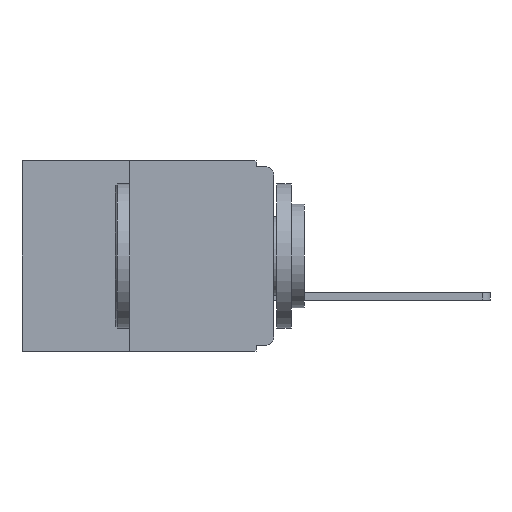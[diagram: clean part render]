
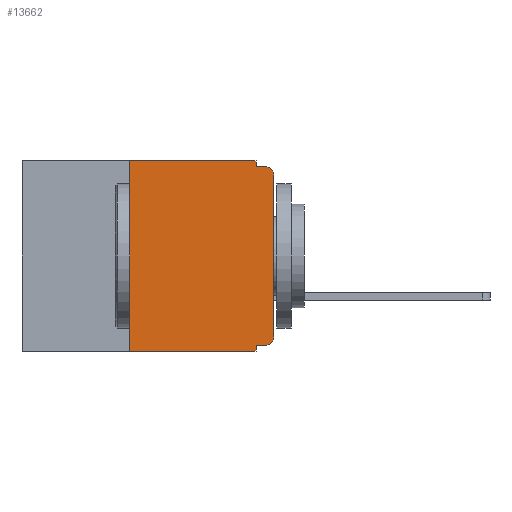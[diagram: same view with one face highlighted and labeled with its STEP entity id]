
A CAD part, left-side view. The second image highlights one B-rep face of the part: STEP entity #13662.
In plain terms, the highlighted planar face has unit normal (-1, 0, 0).
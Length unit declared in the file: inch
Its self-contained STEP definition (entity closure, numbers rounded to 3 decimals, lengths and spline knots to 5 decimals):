
#627 = CARTESIAN_POINT ( 'NONE',  ( 0., 0.031, 0. ) ) ;
#787 = ORIENTED_EDGE ( 'NONE', *, *, #3188, .F. ) ;
#835 = VECTOR ( 'NONE', #8509, 39.37008 ) ;
#1002 = DIRECTION ( 'NONE',  ( 0., 0., 1. ) ) ;
#1035 = CARTESIAN_POINT ( 'NONE',  ( 0., 0.25, 0. ) ) ;
#1057 = VECTOR ( 'NONE', #4462, 39.37008 ) ;
#1366 = CARTESIAN_POINT ( 'NONE',  ( 0., 0., -0.305 ) ) ;
#1656 = CARTESIAN_POINT ( 'NONE',  ( 0., 0.25, -0.33 ) ) ;
#2349 = CARTESIAN_POINT ( 'NONE',  ( 0., 0.031, -0.32 ) ) ;
#2461 = EDGE_CURVE ( 'NONE', #2758, #8635, #11873, .T. ) ;
#2539 = ORIENTED_EDGE ( 'NONE', *, *, #2461, .T. ) ;
#2572 = EDGE_CURVE ( 'NONE', #6670, #8470, #6861, .T. ) ;
#2703 = VERTEX_POINT ( 'NONE', #13685 ) ;
#2758 = VERTEX_POINT ( 'NONE', #6891 ) ;
#2934 = PLANE ( 'NONE',  #12298 ) ;
#3059 = EDGE_CURVE ( 'NONE', #6110, #9530, #4142, .T. ) ;
#3188 = EDGE_CURVE ( 'NONE', #2758, #6728, #3935, .T. ) ;
#3466 = EDGE_CURVE ( 'NONE', #2703, #6555, #9081, .T. ) ;
#3590 = EDGE_CURVE ( 'NONE', #10843, #6110, #10509, .T. ) ;
#3658 = AXIS2_PLACEMENT_3D ( 'NONE', #7960, #7852, #7808 ) ;
#3788 = EDGE_CURVE ( 'NONE', #8470, #9530, #9719, .T. ) ;
#3797 = ORIENTED_EDGE ( 'NONE', *, *, #4057, .F. ) ;
#3935 = LINE ( 'NONE', #1656, #12425 ) ;
#3991 = ORIENTED_EDGE ( 'NONE', *, *, #3466, .F. ) ;
#4057 = EDGE_CURVE ( 'NONE', #6555, #8635, #12536, .T. ) ;
#4110 = DIRECTION ( 'NONE',  ( 1., 0., 0. ) ) ;
#4142 = LINE ( 'NONE', #4792, #7203 ) ;
#4197 = DIRECTION ( 'NONE',  ( 0., -1., 0. ) ) ;
#4209 = EDGE_CURVE ( 'NONE', #2703, #6670, #4679, .T. ) ;
#4229 = ORIENTED_EDGE ( 'NONE', *, *, #4209, .T. ) ;
#4462 = DIRECTION ( 'NONE',  ( 0., 0., -1. ) ) ;
#4679 = CIRCLE ( 'NONE', #8775, 0.015 ) ;
#4792 = CARTESIAN_POINT ( 'NONE',  ( 0., 0., -0.01 ) ) ;
#5159 = ORIENTED_EDGE ( 'NONE', *, *, #3788, .T. ) ;
#5355 = LINE ( 'NONE', #10826, #10720 ) ;
#5729 = EDGE_CURVE ( 'NONE', #6728, #10843, #5355, .T. ) ;
#5818 = VECTOR ( 'NONE', #6712, 39.37008 ) ;
#6037 = DIRECTION ( 'NONE',  ( 0., 0., 1. ) ) ;
#6110 = VERTEX_POINT ( 'NONE', #6798 ) ;
#6408 = ORIENTED_EDGE ( 'NONE', *, *, #3059, .F. ) ;
#6555 = VERTEX_POINT ( 'NONE', #2349 ) ;
#6636 = CARTESIAN_POINT ( 'NONE',  ( 0., 0.031, -0.33 ) ) ;
#6651 = CARTESIAN_POINT ( 'NONE',  ( 0., 0., -0.32 ) ) ;
#6670 = VERTEX_POINT ( 'NONE', #1366 ) ;
#6712 = DIRECTION ( 'NONE',  ( 0., 1., 0. ) ) ;
#6728 = VERTEX_POINT ( 'NONE', #1035 ) ;
#6798 = CARTESIAN_POINT ( 'NONE',  ( 0., 0.031, -0.01 ) ) ;
#6861 = LINE ( 'NONE', #12198, #12288 ) ;
#6891 = CARTESIAN_POINT ( 'NONE',  ( 0., 0.25, -0.33 ) ) ;
#7001 = CARTESIAN_POINT ( 'NONE',  ( 0., 0.031, 0. ) ) ;
#7203 = VECTOR ( 'NONE', #4197, 39.37008 ) ;
#7528 = CARTESIAN_POINT ( 'NONE',  ( 0., 0.437, 0. ) ) ;
#7808 = DIRECTION ( 'NONE',  ( 0., 0., -1. ) ) ;
#7852 = DIRECTION ( 'NONE',  ( -1., 0., 0. ) ) ;
#7942 = CARTESIAN_POINT ( 'NONE',  ( 0., 0.015, -0.01 ) ) ;
#7960 = CARTESIAN_POINT ( 'NONE',  ( 0., 0.015, -0.025 ) ) ;
#8470 = VERTEX_POINT ( 'NONE', #9683 ) ;
#8509 = DIRECTION ( 'NONE',  ( 0., 0., -1. ) ) ;
#8635 = VERTEX_POINT ( 'NONE', #6636 ) ;
#8775 = AXIS2_PLACEMENT_3D ( 'NONE', #11501, #11473, #11470 ) ;
#8936 = VECTOR ( 'NONE', #13142, 39.37008 ) ;
#9081 = LINE ( 'NONE', #6651, #5818 ) ;
#9250 = CARTESIAN_POINT ( 'NONE',  ( 0., 0.031, -0.33 ) ) ;
#9530 = VERTEX_POINT ( 'NONE', #7942 ) ;
#9683 = CARTESIAN_POINT ( 'NONE',  ( 0., 0., -0.025 ) ) ;
#9719 = CIRCLE ( 'NONE', #3658, 0.015 ) ;
#9960 = ORIENTED_EDGE ( 'NONE', *, *, #3590, .F. ) ;
#9985 = EDGE_LOOP ( 'NONE', ( #12767, #5159, #6408, #9960, #13022, #787, #2539, #3797, #3991, #4229 ) ) ;
#10509 = LINE ( 'NONE', #627, #1057 ) ;
#10720 = VECTOR ( 'NONE', #10768, 39.37008 ) ;
#10768 = DIRECTION ( 'NONE',  ( 0., -1., 0. ) ) ;
#10826 = CARTESIAN_POINT ( 'NONE',  ( 0., 0.437, 0. ) ) ;
#10843 = VERTEX_POINT ( 'NONE', #7001 ) ;
#11470 = DIRECTION ( 'NONE',  ( 0., 0., -1. ) ) ;
#11473 = DIRECTION ( 'NONE',  ( -1., 0., 0. ) ) ;
#11501 = CARTESIAN_POINT ( 'NONE',  ( 0., 0.015, -0.305 ) ) ;
#11661 = DIRECTION ( 'NONE',  ( 0., 0., -1. ) ) ;
#11842 = FACE_OUTER_BOUND ( 'NONE', #9985, .T. ) ;
#11873 = LINE ( 'NONE', #12252, #8936 ) ;
#12198 = CARTESIAN_POINT ( 'NONE',  ( 0., 0., 0. ) ) ;
#12252 = CARTESIAN_POINT ( 'NONE',  ( 0., 0.437, -0.33 ) ) ;
#12288 = VECTOR ( 'NONE', #6037, 39.37008 ) ;
#12298 = AXIS2_PLACEMENT_3D ( 'NONE', #7528, #4110, #11661 ) ;
#12425 = VECTOR ( 'NONE', #1002, 39.37008 ) ;
#12536 = LINE ( 'NONE', #9250, #835 ) ;
#12767 = ORIENTED_EDGE ( 'NONE', *, *, #2572, .T. ) ;
#13022 = ORIENTED_EDGE ( 'NONE', *, *, #5729, .F. ) ;
#13142 = DIRECTION ( 'NONE',  ( 0., -1., 0. ) ) ;
#13662 = ADVANCED_FACE ( 'NONE', ( #11842 ), #2934, .F. ) ;
#13685 = CARTESIAN_POINT ( 'NONE',  ( 0., 0.015, -0.32 ) ) ;
